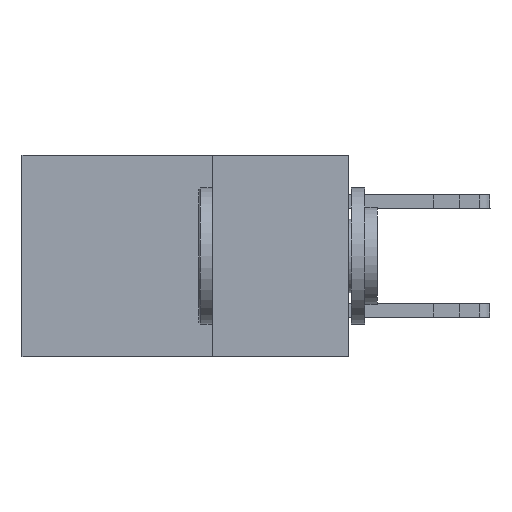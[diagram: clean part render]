
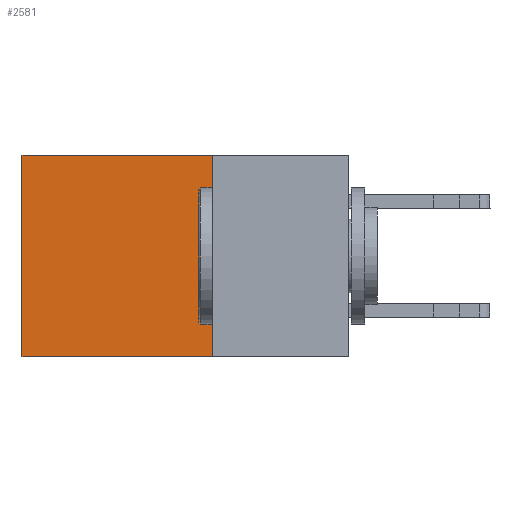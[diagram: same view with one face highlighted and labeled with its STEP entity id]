
A CAD part, left-side view. The second image highlights one B-rep face of the part: STEP entity #2581.
In plain terms, the highlighted planar face has unit normal (-1, 0, 0).
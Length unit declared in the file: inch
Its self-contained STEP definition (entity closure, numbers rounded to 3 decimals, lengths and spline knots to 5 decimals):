
#38 = CARTESIAN_POINT ( 'NONE',  ( 0.2615, 0.25, -0.37 ) ) ;
#256 = DIRECTION ( 'NONE',  ( 0., 0., -1. ) ) ;
#546 = VECTOR ( 'NONE', #10020, 39.37008 ) ;
#1259 = PLANE ( 'NONE',  #9410 ) ;
#1779 = ORIENTED_EDGE ( 'NONE', *, *, #8171, .F. ) ;
#1853 = LINE ( 'NONE', #8179, #10907 ) ;
#1994 = VERTEX_POINT ( 'NONE', #9843 ) ;
#2151 = EDGE_CURVE ( 'NONE', #10479, #9990, #1853, .T. ) ;
#2378 = ORIENTED_EDGE ( 'NONE', *, *, #2151, .T. ) ;
#2581 = ADVANCED_FACE ( 'NONE', ( #8364 ), #1259, .F. ) ;
#2991 = DIRECTION ( 'NONE',  ( 1., 0., 0. ) ) ;
#3067 = DIRECTION ( 'NONE',  ( 0., 1., 0. ) ) ;
#3987 = VECTOR ( 'NONE', #3067, 39.37008 ) ;
#4436 = CARTESIAN_POINT ( 'NONE',  ( 0.2615, 0.25, 0. ) ) ;
#5143 = EDGE_CURVE ( 'NONE', #1994, #10479, #6209, .T. ) ;
#5198 = DIRECTION ( 'NONE',  ( 0., 1., 0. ) ) ;
#5465 = DIRECTION ( 'NONE',  ( 0., 0., -1. ) ) ;
#6209 = LINE ( 'NONE', #4436, #10923 ) ;
#6719 = EDGE_LOOP ( 'NONE', ( #2378, #11669, #1779, #8521 ) ) ;
#7246 = CARTESIAN_POINT ( 'NONE',  ( 0.2615, 0.25, -0.37 ) ) ;
#7536 = CARTESIAN_POINT ( 'NONE',  ( 0.2615, 0.25, -0.37 ) ) ;
#7734 = VERTEX_POINT ( 'NONE', #38 ) ;
#8171 = EDGE_CURVE ( 'NONE', #1994, #7734, #9068, .T. ) ;
#8179 = CARTESIAN_POINT ( 'NONE',  ( 0.2615, 0.6, -0.37 ) ) ;
#8364 = FACE_OUTER_BOUND ( 'NONE', #6719, .T. ) ;
#8521 = ORIENTED_EDGE ( 'NONE', *, *, #5143, .T. ) ;
#8555 = CARTESIAN_POINT ( 'NONE',  ( 0.2615, 0.25, -0.37 ) ) ;
#8601 = CARTESIAN_POINT ( 'NONE',  ( 0.2615, 0.6, -0.37 ) ) ;
#9068 = LINE ( 'NONE', #7246, #546 ) ;
#9203 = LINE ( 'NONE', #8555, #3987 ) ;
#9410 = AXIS2_PLACEMENT_3D ( 'NONE', #7536, #2991, #256 ) ;
#9755 = EDGE_CURVE ( 'NONE', #7734, #9990, #9203, .T. ) ;
#9843 = CARTESIAN_POINT ( 'NONE',  ( 0.2615, 0.25, 0. ) ) ;
#9990 = VERTEX_POINT ( 'NONE', #8601 ) ;
#10020 = DIRECTION ( 'NONE',  ( 0., 0., -1. ) ) ;
#10479 = VERTEX_POINT ( 'NONE', #11059 ) ;
#10907 = VECTOR ( 'NONE', #5465, 39.37008 ) ;
#10923 = VECTOR ( 'NONE', #5198, 39.37008 ) ;
#11059 = CARTESIAN_POINT ( 'NONE',  ( 0.2615, 0.6, 0. ) ) ;
#11669 = ORIENTED_EDGE ( 'NONE', *, *, #9755, .F. ) ;
